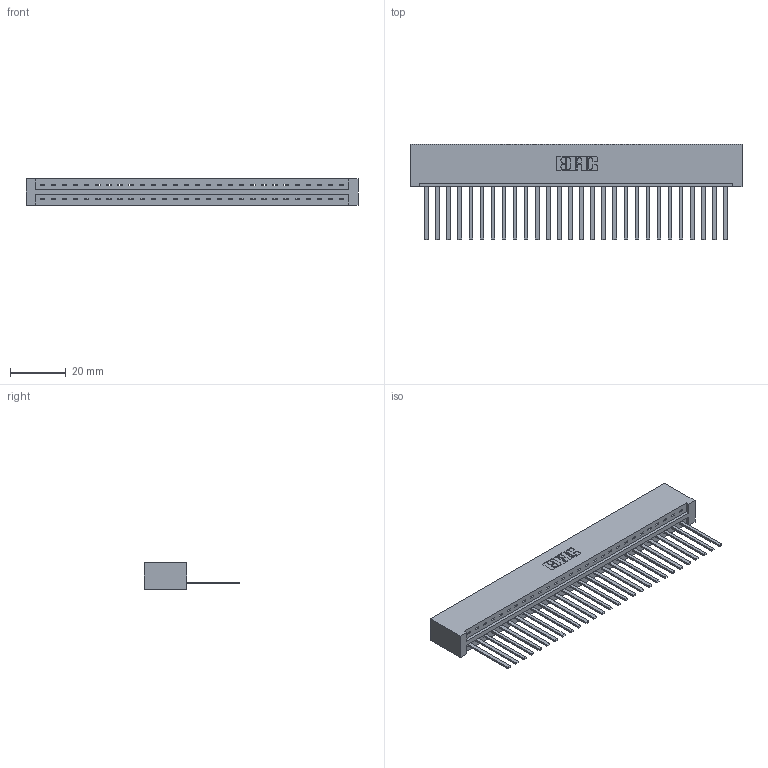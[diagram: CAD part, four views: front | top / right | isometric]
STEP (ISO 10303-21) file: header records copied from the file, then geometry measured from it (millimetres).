
FILE_DESCRIPTION (( 'STEP AP203' ), '1' );
FILE_NAME ('387-028-544-101.STEP', '2018-09-16T21:59:27', ( '' ), ( '' ), 'SwSTEP 2.0', 'SolidWorks 2016', '' );
FILE_SCHEMA (( 'CONFIG_CONTROL_DESIGN' ));
Length unit declared in the file: inch
Products named in the file (3): 337 Part_No Mounting Lugs; 345-292-001_345-293-144; 387-028-544-101
Assembly tree (29 placements, depth 2):
  387-028-544-101
    337 Part_No Mounting Lugs
    345-292-001_345-293-144  x28
Bounding box: 118.82 x 34.3 x 9.4 mm (x, y, z)
Volume: 13237.3 mm3; surface area: 14649.2 mm2
Topology: 29 solids, 29 shells, 1674 faces, 5047 edges, 3326 vertices
Faces by surface type: plane 1242, cylinder 432
Entity records: 22163 total; most frequent: CARTESIAN_POINT 3866, ORIENTED_EDGE 3830, DIRECTION 3271, EDGE_CURVE 1915, LINE 1799, VECTOR 1799, VERTEX_POINT 1274, AXIS2_PLACEMENT_3D 736
